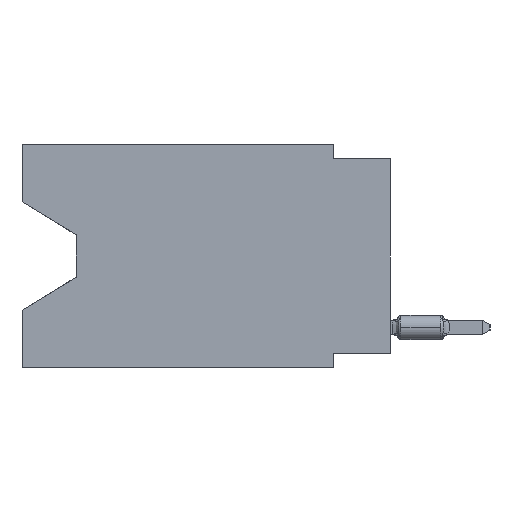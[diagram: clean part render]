
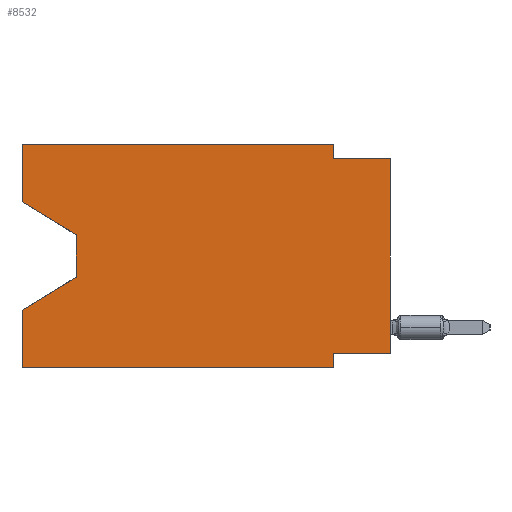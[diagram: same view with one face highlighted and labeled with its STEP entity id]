
A CAD part, left-side view. The second image highlights one B-rep face of the part: STEP entity #8532.
In plain terms, the highlighted planar face has unit normal (-1, 0, 0).
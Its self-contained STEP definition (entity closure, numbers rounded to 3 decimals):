
#274 = CARTESIAN_POINT ( 'NONE',  ( 0., 13.97, -4.013 ) ) ;
#299 = DIRECTION ( 'NONE',  ( 0., -1., 0. ) ) ;
#703 = CARTESIAN_POINT ( 'NONE',  ( 0., 16.383, 0. ) ) ;
#745 = VECTOR ( 'NONE', #7998, 1000. ) ;
#866 = EDGE_CURVE ( 'NONE', #4357, #15448, #27441, .T. ) ;
#1258 = VECTOR ( 'NONE', #25854, 1000. ) ;
#1580 = VERTEX_POINT ( 'NONE', #31026 ) ;
#1808 = DIRECTION ( 'NONE',  ( 0., 0., 1. ) ) ;
#2420 = EDGE_CURVE ( 'NONE', #19229, #40592, #4780, .T. ) ;
#4357 = VERTEX_POINT ( 'NONE', #29975 ) ;
#4780 = LINE ( 'NONE', #37996, #36044 ) ;
#4841 = LINE ( 'NONE', #38056, #31901 ) ;
#5087 = DIRECTION ( 'NONE',  ( 0., 0., 1. ) ) ;
#5176 = VECTOR ( 'NONE', #40127, 1000. ) ;
#5421 = CARTESIAN_POINT ( 'NONE',  ( 0., 2.54, -0.635 ) ) ;
#5547 = CARTESIAN_POINT ( 'NONE',  ( 0., 16.383, -2.546 ) ) ;
#5708 = ORIENTED_EDGE ( 'NONE', *, *, #13582, .F. ) ;
#5943 = ORIENTED_EDGE ( 'NONE', *, *, #30206, .F. ) ;
#6864 = CARTESIAN_POINT ( 'NONE',  ( 0., 2.54, -9.271 ) ) ;
#7998 = DIRECTION ( 'NONE',  ( 0., -1., 0. ) ) ;
#8048 = DIRECTION ( 'NONE',  ( 0., 0., -1. ) ) ;
#8532 = ADVANCED_FACE ( 'NONE', ( #30014 ), #17648, .F. ) ;
#8611 = VECTOR ( 'NONE', #299, 1000. ) ;
#8791 = EDGE_CURVE ( 'NONE', #40970, #1580, #9571, .T. ) ;
#9571 = LINE ( 'NONE', #38878, #1258 ) ;
#10256 = CARTESIAN_POINT ( 'NONE',  ( 0., 16.383, 0. ) ) ;
#10467 = CARTESIAN_POINT ( 'NONE',  ( 0., 16.383, 0. ) ) ;
#10701 = DIRECTION ( 'NONE',  ( 0., 0., -1. ) ) ;
#11167 = CARTESIAN_POINT ( 'NONE',  ( 0., 16.383, 0. ) ) ;
#11188 = VECTOR ( 'NONE', #41318, 1000. ) ;
#11681 = VECTOR ( 'NONE', #5087, 1000. ) ;
#12579 = VERTEX_POINT ( 'NONE', #274 ) ;
#13185 = EDGE_CURVE ( 'NONE', #12579, #33048, #41463, .T. ) ;
#13300 = VECTOR ( 'NONE', #16765, 1000. ) ;
#13582 = EDGE_CURVE ( 'NONE', #40592, #1580, #37736, .T. ) ;
#14306 = CARTESIAN_POINT ( 'NONE',  ( 0., 16.383, -7.36 ) ) ;
#14323 = ORIENTED_EDGE ( 'NONE', *, *, #18032, .F. ) ;
#14785 = DIRECTION ( 'NONE',  ( 0., 0., -1. ) ) ;
#15448 = VERTEX_POINT ( 'NONE', #703 ) ;
#15467 = ORIENTED_EDGE ( 'NONE', *, *, #19779, .T. ) ;
#16765 = DIRECTION ( 'NONE',  ( 0., -1., 0. ) ) ;
#16813 = CARTESIAN_POINT ( 'NONE',  ( 0., 16.383, -9.906 ) ) ;
#16820 = CARTESIAN_POINT ( 'NONE',  ( 0., 2.54, -9.906 ) ) ;
#17648 = PLANE ( 'NONE',  #25466 ) ;
#18032 = EDGE_CURVE ( 'NONE', #15448, #19229, #22841, .T. ) ;
#18749 = VECTOR ( 'NONE', #8048, 1000. ) ;
#18778 = ORIENTED_EDGE ( 'NONE', *, *, #27098, .F. ) ;
#19229 = VERTEX_POINT ( 'NONE', #28992 ) ;
#19779 = EDGE_CURVE ( 'NONE', #19978, #29871, #39172, .T. ) ;
#19978 = VERTEX_POINT ( 'NONE', #20284 ) ;
#20248 = DIRECTION ( 'NONE',  ( 1., 0., 0. ) ) ;
#20284 = CARTESIAN_POINT ( 'NONE',  ( 0., 16.383, -9.906 ) ) ;
#21219 = ORIENTED_EDGE ( 'NONE', *, *, #13185, .T. ) ;
#21361 = VERTEX_POINT ( 'NONE', #6864 ) ;
#21484 = CARTESIAN_POINT ( 'NONE',  ( 0., 13.97, -4.013 ) ) ;
#22079 = EDGE_CURVE ( 'NONE', #33048, #25446, #26875, .T. ) ;
#22338 = ORIENTED_EDGE ( 'NONE', *, *, #36120, .T. ) ;
#22536 = ORIENTED_EDGE ( 'NONE', *, *, #8791, .T. ) ;
#22841 = LINE ( 'NONE', #10467, #13300 ) ;
#23010 = ORIENTED_EDGE ( 'NONE', *, *, #2420, .F. ) ;
#24795 = LINE ( 'NONE', #31327, #11188 ) ;
#25059 = VECTOR ( 'NONE', #41396, 1000. ) ;
#25446 = VERTEX_POINT ( 'NONE', #14306 ) ;
#25466 = AXIS2_PLACEMENT_3D ( 'NONE', #10256, #20248, #10701 ) ;
#25566 = VECTOR ( 'NONE', #39767, 1000. ) ;
#25854 = DIRECTION ( 'NONE',  ( 0., 0., 1. ) ) ;
#26875 = LINE ( 'NONE', #39922, #5176 ) ;
#27098 = EDGE_CURVE ( 'NONE', #40970, #21361, #24795, .T. ) ;
#27441 = LINE ( 'NONE', #11167, #11681 ) ;
#27941 = LINE ( 'NONE', #5547, #25059 ) ;
#28992 = CARTESIAN_POINT ( 'NONE',  ( 0., 2.54, 0. ) ) ;
#29358 = ORIENTED_EDGE ( 'NONE', *, *, #866, .F. ) ;
#29871 = VERTEX_POINT ( 'NONE', #16820 ) ;
#29975 = CARTESIAN_POINT ( 'NONE',  ( 0., 16.383, -2.546 ) ) ;
#30014 = FACE_OUTER_BOUND ( 'NONE', #31082, .T. ) ;
#30206 = EDGE_CURVE ( 'NONE', #21361, #29871, #30216, .T. ) ;
#30216 = LINE ( 'NONE', #33687, #25566 ) ;
#31026 = CARTESIAN_POINT ( 'NONE',  ( 0., 0., -0.635 ) ) ;
#31082 = EDGE_LOOP ( 'NONE', ( #22338, #21219, #37051, #36244, #15467, #5943, #18778, #22536, #5708, #23010, #14323, #29358 ) ) ;
#31327 = CARTESIAN_POINT ( 'NONE',  ( 0., 0., -9.271 ) ) ;
#31901 = VECTOR ( 'NONE', #1808, 1000. ) ;
#31930 = EDGE_CURVE ( 'NONE', #19978, #25446, #4841, .T. ) ;
#33048 = VERTEX_POINT ( 'NONE', #35360 ) ;
#33687 = CARTESIAN_POINT ( 'NONE',  ( 0., 2.54, -9.906 ) ) ;
#34026 = CARTESIAN_POINT ( 'NONE',  ( 0., 0., -0.635 ) ) ;
#35360 = CARTESIAN_POINT ( 'NONE',  ( 0., 13.97, -5.893 ) ) ;
#36044 = VECTOR ( 'NONE', #14785, 1000. ) ;
#36120 = EDGE_CURVE ( 'NONE', #4357, #12579, #27941, .T. ) ;
#36244 = ORIENTED_EDGE ( 'NONE', *, *, #31930, .F. ) ;
#37051 = ORIENTED_EDGE ( 'NONE', *, *, #22079, .T. ) ;
#37736 = LINE ( 'NONE', #34026, #745 ) ;
#37996 = CARTESIAN_POINT ( 'NONE',  ( 0., 2.54, 0. ) ) ;
#38056 = CARTESIAN_POINT ( 'NONE',  ( 0., 16.383, 0. ) ) ;
#38878 = CARTESIAN_POINT ( 'NONE',  ( 0., 0., 0. ) ) ;
#39172 = LINE ( 'NONE', #16813, #8611 ) ;
#39767 = DIRECTION ( 'NONE',  ( 0., 0., -1. ) ) ;
#39922 = CARTESIAN_POINT ( 'NONE',  ( 0., 13.97, -5.893 ) ) ;
#40127 = DIRECTION ( 'NONE',  ( 0., 0.855, -0.519 ) ) ;
#40592 = VERTEX_POINT ( 'NONE', #5421 ) ;
#40970 = VERTEX_POINT ( 'NONE', #41427 ) ;
#41318 = DIRECTION ( 'NONE',  ( 0., 1., 0. ) ) ;
#41396 = DIRECTION ( 'NONE',  ( 0., -0.855, -0.519 ) ) ;
#41427 = CARTESIAN_POINT ( 'NONE',  ( 0., 0., -9.271 ) ) ;
#41463 = LINE ( 'NONE', #21484, #18749 ) ;
